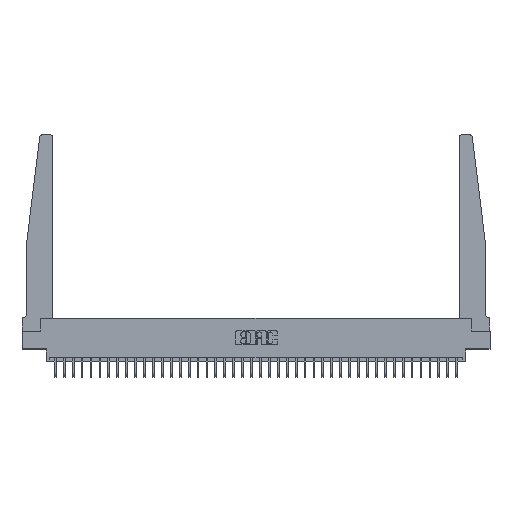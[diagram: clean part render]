
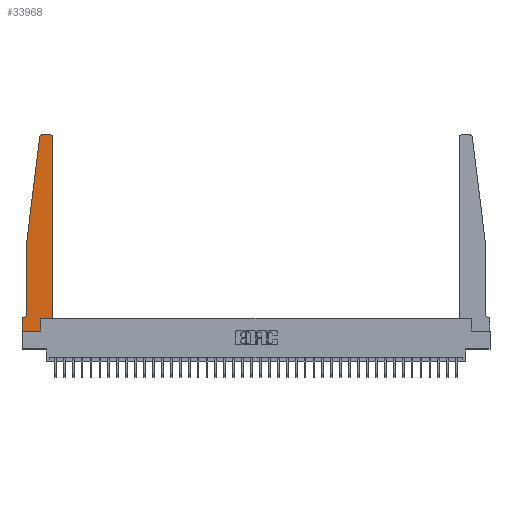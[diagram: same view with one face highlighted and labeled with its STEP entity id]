
A CAD part, top view. The second image highlights one B-rep face of the part: STEP entity #33968.
In plain terms, the highlighted planar face has unit normal (0, 0, 1).
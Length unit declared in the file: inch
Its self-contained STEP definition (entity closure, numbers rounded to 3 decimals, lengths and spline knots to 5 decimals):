
#653 = CARTESIAN_POINT ( 'NONE',  ( 0.2605, 0., 0.37 ) ) ;
#1875 = CARTESIAN_POINT ( 'NONE',  ( 0.065, 1.25, 0.37 ) ) ;
#2094 = CARTESIAN_POINT ( 'NONE',  ( 0.24675, 2.72367, 0.37 ) ) ;
#2248 = DIRECTION ( 'NONE',  ( 0., 0., -1. ) ) ;
#2375 = EDGE_CURVE ( 'NONE', #9330, #21466, #25847, .T. ) ;
#2796 = EDGE_CURVE ( 'NONE', #4918, #12446, #10933, .T. ) ;
#3322 = CARTESIAN_POINT ( 'NONE',  ( 0.395, 2.75, 0.37 ) ) ;
#4071 = CARTESIAN_POINT ( 'NONE',  ( 0.2605, 0.18, 0.37 ) ) ;
#4113 = DIRECTION ( 'NONE',  ( -1., 0., 0. ) ) ;
#4727 = CARTESIAN_POINT ( 'NONE',  ( 0.425, 2.72, 0.37 ) ) ;
#4884 = VECTOR ( 'NONE', #4113, 39.37008 ) ;
#4918 = VERTEX_POINT ( 'NONE', #4071 ) ;
#5335 = CARTESIAN_POINT ( 'NONE',  ( 0.065, 0.2375, 0.37 ) ) ;
#5557 = EDGE_CURVE ( 'NONE', #18031, #5815, #16900, .T. ) ;
#5815 = VERTEX_POINT ( 'NONE', #1875 ) ;
#7017 = VECTOR ( 'NONE', #35366, 39.37008 ) ;
#7224 = LINE ( 'NONE', #8115, #35708 ) ;
#7444 = AXIS2_PLACEMENT_3D ( 'NONE', #21039, #23362, #18002 ) ;
#8115 = CARTESIAN_POINT ( 'NONE',  ( 0.2605, 0.18, 0.37 ) ) ;
#8393 = CARTESIAN_POINT ( 'NONE',  ( 0.27653, 2.72, 0.37 ) ) ;
#8720 = ORIENTED_EDGE ( 'NONE', *, *, #2796, .T. ) ;
#9330 = VERTEX_POINT ( 'NONE', #5335 ) ;
#9513 = ORIENTED_EDGE ( 'NONE', *, *, #2375, .T. ) ;
#10933 = LINE ( 'NONE', #31042, #29295 ) ;
#11257 = DIRECTION ( 'NONE',  ( 1., 0., 0. ) ) ;
#11481 = CARTESIAN_POINT ( 'NONE',  ( 0.395, 2.72, 0.37 ) ) ;
#11870 = LINE ( 'NONE', #28450, #23729 ) ;
#12291 = VERTEX_POINT ( 'NONE', #15016 ) ;
#12446 = VERTEX_POINT ( 'NONE', #24987 ) ;
#12932 = ORIENTED_EDGE ( 'NONE', *, *, #19784, .T. ) ;
#13112 = VERTEX_POINT ( 'NONE', #20001 ) ;
#13322 = ORIENTED_EDGE ( 'NONE', *, *, #31283, .T. ) ;
#13377 = AXIS2_PLACEMENT_3D ( 'NONE', #19022, #2248, #32922 ) ;
#14438 = EDGE_CURVE ( 'NONE', #12291, #23707, #29076, .T. ) ;
#14806 = EDGE_CURVE ( 'NONE', #23707, #4918, #7224, .T. ) ;
#14866 = CARTESIAN_POINT ( 'NONE',  ( 0.27653, 2.75, 0.37 ) ) ;
#15016 = CARTESIAN_POINT ( 'NONE',  ( 0., 0., 0.37 ) ) ;
#15202 = AXIS2_PLACEMENT_3D ( 'NONE', #11481, #22988, #17115 ) ;
#15470 = VECTOR ( 'NONE', #33128, 39.37008 ) ;
#15913 = ORIENTED_EDGE ( 'NONE', *, *, #33279, .T. ) ;
#15976 = LINE ( 'NONE', #20037, #21240 ) ;
#16900 = LINE ( 'NONE', #16987, #34372 ) ;
#16987 = CARTESIAN_POINT ( 'NONE',  ( 0.065, 1.25, 0.37 ) ) ;
#17115 = DIRECTION ( 'NONE',  ( 1., 0., 0. ) ) ;
#17122 = LINE ( 'NONE', #21206, #7017 ) ;
#18002 = DIRECTION ( 'NONE',  ( 1., 0., 0. ) ) ;
#18031 = VERTEX_POINT ( 'NONE', #2094 ) ;
#18874 = FACE_OUTER_BOUND ( 'NONE', #20380, .T. ) ;
#19022 = CARTESIAN_POINT ( 'NONE',  ( 0.015, 0.2375, 0.37 ) ) ;
#19784 = EDGE_CURVE ( 'NONE', #21466, #13112, #31980, .T. ) ;
#20001 = CARTESIAN_POINT ( 'NONE',  ( 0., 0.1875, 0.37 ) ) ;
#20037 = CARTESIAN_POINT ( 'NONE',  ( 0.065, 1.25, 0.37 ) ) ;
#20372 = ORIENTED_EDGE ( 'NONE', *, *, #24881, .T. ) ;
#20380 = EDGE_LOOP ( 'NONE', ( #15913, #20372, #35479, #13322, #9513, #12932, #36068, #25385, #34851, #8720, #21972, #28239 ) ) ;
#21039 = CARTESIAN_POINT ( 'NONE',  ( 0., 0.1875, 0.37 ) ) ;
#21206 = CARTESIAN_POINT ( 'NONE',  ( 0.425, 0.18, 0.37 ) ) ;
#21240 = VECTOR ( 'NONE', #25311, 39.37008 ) ;
#21466 = VERTEX_POINT ( 'NONE', #27226 ) ;
#21972 = ORIENTED_EDGE ( 'NONE', *, *, #22613, .T. ) ;
#22613 = EDGE_CURVE ( 'NONE', #12446, #34883, #17122, .T. ) ;
#22929 = EDGE_CURVE ( 'NONE', #34883, #33831, #25823, .T. ) ;
#22988 = DIRECTION ( 'NONE',  ( 0., 0., 1. ) ) ;
#23362 = DIRECTION ( 'NONE',  ( 0., 0., 1. ) ) ;
#23707 = VERTEX_POINT ( 'NONE', #653 ) ;
#23729 = VECTOR ( 'NONE', #31562, 39.37008 ) ;
#23923 = VECTOR ( 'NONE', #23939, 39.37008 ) ;
#23939 = DIRECTION ( 'NONE',  ( 0., -1., 0. ) ) ;
#24451 = CARTESIAN_POINT ( 'NONE',  ( 0., 0., 0.37 ) ) ;
#24881 = EDGE_CURVE ( 'NONE', #25630, #18031, #30042, .T. ) ;
#24987 = CARTESIAN_POINT ( 'NONE',  ( 0.425, 0.18, 0.37 ) ) ;
#25231 = LINE ( 'NONE', #35166, #23923 ) ;
#25253 = EDGE_CURVE ( 'NONE', #13112, #12291, #25231, .T. ) ;
#25311 = DIRECTION ( 'NONE',  ( 0., -1., 0. ) ) ;
#25385 = ORIENTED_EDGE ( 'NONE', *, *, #14438, .T. ) ;
#25630 = VERTEX_POINT ( 'NONE', #14866 ) ;
#25823 = CIRCLE ( 'NONE', #15202, 0.03 ) ;
#25847 = CIRCLE ( 'NONE', #13377, 0.05 ) ;
#27219 = DIRECTION ( 'NONE',  ( 0., 1., 0. ) ) ;
#27226 = CARTESIAN_POINT ( 'NONE',  ( 0.015, 0.1875, 0.37 ) ) ;
#28239 = ORIENTED_EDGE ( 'NONE', *, *, #22929, .T. ) ;
#28450 = CARTESIAN_POINT ( 'NONE',  ( 0.25, 2.75, 0.37 ) ) ;
#29076 = LINE ( 'NONE', #24451, #15470 ) ;
#29295 = VECTOR ( 'NONE', #33508, 39.37008 ) ;
#30042 = CIRCLE ( 'NONE', #31594, 0.03 ) ;
#30416 = DIRECTION ( 'NONE',  ( 0., 0., 1. ) ) ;
#31042 = CARTESIAN_POINT ( 'NONE',  ( 0.425, 0.18, 0.37 ) ) ;
#31283 = EDGE_CURVE ( 'NONE', #5815, #9330, #15976, .T. ) ;
#31562 = DIRECTION ( 'NONE',  ( -1., 0., 0. ) ) ;
#31594 = AXIS2_PLACEMENT_3D ( 'NONE', #8393, #30416, #11257 ) ;
#31653 = PLANE ( 'NONE',  #7444 ) ;
#31980 = LINE ( 'NONE', #32346, #4884 ) ;
#32346 = CARTESIAN_POINT ( 'NONE',  ( 0.065, 0.1875, 0.37 ) ) ;
#32922 = DIRECTION ( 'NONE',  ( -1., 0., 0. ) ) ;
#33128 = DIRECTION ( 'NONE',  ( 1., 0., 0. ) ) ;
#33279 = EDGE_CURVE ( 'NONE', #33831, #25630, #11870, .T. ) ;
#33508 = DIRECTION ( 'NONE',  ( 1., 0., 0. ) ) ;
#33592 = DIRECTION ( 'NONE',  ( -0.122, -0.992, 0. ) ) ;
#33831 = VERTEX_POINT ( 'NONE', #3322 ) ;
#33968 = ADVANCED_FACE ( 'NONE', ( #18874 ), #31653, .T. ) ;
#34372 = VECTOR ( 'NONE', #33592, 39.37008 ) ;
#34851 = ORIENTED_EDGE ( 'NONE', *, *, #14806, .T. ) ;
#34883 = VERTEX_POINT ( 'NONE', #4727 ) ;
#35166 = CARTESIAN_POINT ( 'NONE',  ( 0., 0., 0.37 ) ) ;
#35366 = DIRECTION ( 'NONE',  ( 0., 1., 0. ) ) ;
#35479 = ORIENTED_EDGE ( 'NONE', *, *, #5557, .T. ) ;
#35708 = VECTOR ( 'NONE', #27219, 39.37008 ) ;
#36068 = ORIENTED_EDGE ( 'NONE', *, *, #25253, .T. ) ;
